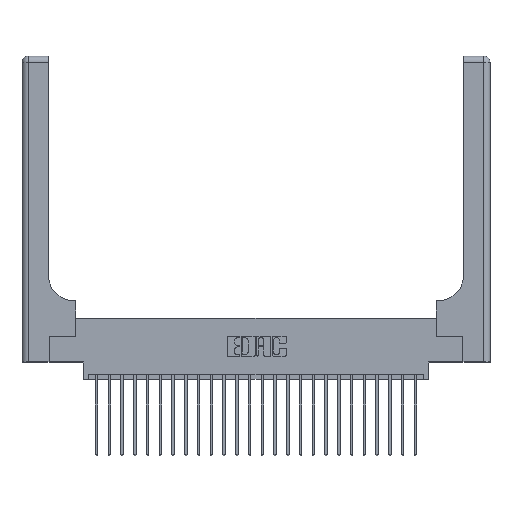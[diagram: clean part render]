
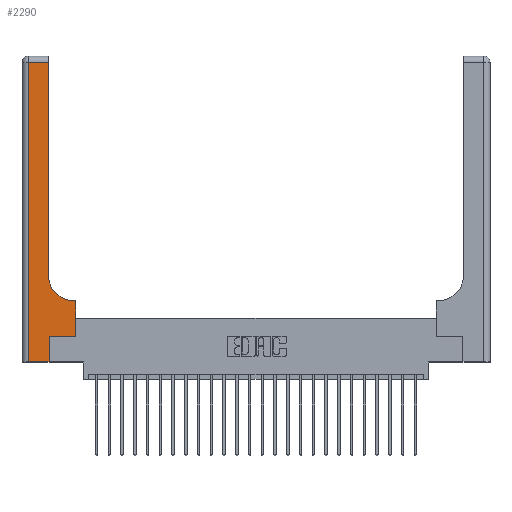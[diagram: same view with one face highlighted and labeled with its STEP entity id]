
A CAD part, top view. The second image highlights one B-rep face of the part: STEP entity #2290.
In plain terms, the highlighted planar face has unit normal (0, 0, 1).
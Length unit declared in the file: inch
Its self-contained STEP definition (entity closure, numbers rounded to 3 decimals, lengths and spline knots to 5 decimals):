
#198 = DIRECTION ( 'NONE',  ( 1., 0., 0. ) ) ;
#239 = EDGE_CURVE ( 'NONE', #23521, #16799, #15904, .T. ) ;
#291 = EDGE_LOOP ( 'NONE', ( #4478, #24592, #1871, #3739, #15681, #24732, #485, #9673, #7889 ) ) ;
#323 = CARTESIAN_POINT ( 'NONE',  ( 0.528, 0.25, 0.37 ) ) ;
#444 = DIRECTION ( 'NONE',  ( -1., 0., 0. ) ) ;
#485 = ORIENTED_EDGE ( 'NONE', *, *, #17628, .T. ) ;
#491 = VECTOR ( 'NONE', #2078, 39.37008 ) ;
#768 = VERTEX_POINT ( 'NONE', #23252 ) ;
#854 = VERTEX_POINT ( 'NONE', #15691 ) ;
#862 = VECTOR ( 'NONE', #1539, 39.37008 ) ;
#1539 = DIRECTION ( 'NONE',  ( 0., 1., 0. ) ) ;
#1871 = ORIENTED_EDGE ( 'NONE', *, *, #14833, .T. ) ;
#2078 = DIRECTION ( 'NONE',  ( -1., 0., 0. ) ) ;
#2208 = CARTESIAN_POINT ( 'NONE',  ( 0.26, 0.6, 0.37 ) ) ;
#2290 = ADVANCED_FACE ( 'NONE', ( #17713 ), #2577, .F. ) ;
#2577 = PLANE ( 'NONE',  #14267 ) ;
#2630 = DIRECTION ( 'NONE',  ( 0., 1., 0. ) ) ;
#2984 = VECTOR ( 'NONE', #18161, 39.37008 ) ;
#3313 = VERTEX_POINT ( 'NONE', #3634 ) ;
#3634 = CARTESIAN_POINT ( 'NONE',  ( 0.26, 2.94, 0.37 ) ) ;
#3709 = CARTESIAN_POINT ( 'NONE',  ( 0.265, 0., 0.37 ) ) ;
#3739 = ORIENTED_EDGE ( 'NONE', *, *, #14933, .T. ) ;
#3963 = VERTEX_POINT ( 'NONE', #13200 ) ;
#3987 = DIRECTION ( 'NONE',  ( 0., 0., -1. ) ) ;
#4138 = EDGE_CURVE ( 'NONE', #13338, #23521, #16810, .T. ) ;
#4478 = ORIENTED_EDGE ( 'NONE', *, *, #21760, .T. ) ;
#4628 = VERTEX_POINT ( 'NONE', #5416 ) ;
#5118 = EDGE_CURVE ( 'NONE', #854, #22644, #17482, .T. ) ;
#5131 = EDGE_CURVE ( 'NONE', #3313, #4628, #15595, .T. ) ;
#5416 = CARTESIAN_POINT ( 'NONE',  ( 0.06, 2.94, 0.37 ) ) ;
#5643 = CARTESIAN_POINT ( 'NONE',  ( 0.06, 3., 0.37 ) ) ;
#5755 = CARTESIAN_POINT ( 'NONE',  ( 0., 2.94, 0.37 ) ) ;
#6019 = CARTESIAN_POINT ( 'NONE',  ( 0., 0., 0.37 ) ) ;
#6179 = AXIS2_PLACEMENT_3D ( 'NONE', #12033, #23136, #198 ) ;
#7767 = DIRECTION ( 'NONE',  ( 1., 0., 0. ) ) ;
#7889 = ORIENTED_EDGE ( 'NONE', *, *, #22167, .T. ) ;
#8161 = VECTOR ( 'NONE', #8395, 39.37008 ) ;
#8395 = DIRECTION ( 'NONE',  ( 0., 1., 0. ) ) ;
#8538 = LINE ( 'NONE', #19910, #23062 ) ;
#8716 = LINE ( 'NONE', #6019, #21770 ) ;
#8886 = VECTOR ( 'NONE', #24309, 39.37008 ) ;
#9673 = ORIENTED_EDGE ( 'NONE', *, *, #5118, .T. ) ;
#11314 = LINE ( 'NONE', #5643, #8886 ) ;
#12033 = CARTESIAN_POINT ( 'NONE',  ( 0.51, 0.85, 0.37 ) ) ;
#13200 = CARTESIAN_POINT ( 'NONE',  ( 0.26, 0.85, 0.37 ) ) ;
#13338 = VERTEX_POINT ( 'NONE', #3709 ) ;
#13553 = CARTESIAN_POINT ( 'NONE',  ( 0., 3., 0.37 ) ) ;
#14003 = CARTESIAN_POINT ( 'NONE',  ( 0.265, 0.25, 0.37 ) ) ;
#14267 = AXIS2_PLACEMENT_3D ( 'NONE', #13553, #3987, #444 ) ;
#14833 = EDGE_CURVE ( 'NONE', #4628, #768, #11314, .T. ) ;
#14933 = EDGE_CURVE ( 'NONE', #768, #13338, #8716, .T. ) ;
#15595 = LINE ( 'NONE', #5755, #16210 ) ;
#15681 = ORIENTED_EDGE ( 'NONE', *, *, #4138, .T. ) ;
#15691 = CARTESIAN_POINT ( 'NONE',  ( 0.528, 0.6, 0.37 ) ) ;
#15904 = LINE ( 'NONE', #14003, #2984 ) ;
#16210 = VECTOR ( 'NONE', #21137, 39.37008 ) ;
#16799 = VERTEX_POINT ( 'NONE', #323 ) ;
#16810 = LINE ( 'NONE', #18818, #862 ) ;
#17482 = LINE ( 'NONE', #2208, #491 ) ;
#17628 = EDGE_CURVE ( 'NONE', #16799, #854, #8538, .T. ) ;
#17713 = FACE_OUTER_BOUND ( 'NONE', #291, .T. ) ;
#18161 = DIRECTION ( 'NONE',  ( 1., 0., 0. ) ) ;
#18262 = CIRCLE ( 'NONE', #6179, 0.25 ) ;
#18818 = CARTESIAN_POINT ( 'NONE',  ( 0.265, 0., 0.37 ) ) ;
#19479 = CARTESIAN_POINT ( 'NONE',  ( 0.265, 0.25, 0.37 ) ) ;
#19910 = CARTESIAN_POINT ( 'NONE',  ( 0.528, 0.25, 0.37 ) ) ;
#20258 = LINE ( 'NONE', #22393, #8161 ) ;
#21137 = DIRECTION ( 'NONE',  ( -1., 0., 0. ) ) ;
#21213 = CARTESIAN_POINT ( 'NONE',  ( 0.51, 0.6, 0.37 ) ) ;
#21760 = EDGE_CURVE ( 'NONE', #3963, #3313, #20258, .T. ) ;
#21770 = VECTOR ( 'NONE', #7767, 39.37008 ) ;
#22167 = EDGE_CURVE ( 'NONE', #22644, #3963, #18262, .T. ) ;
#22393 = CARTESIAN_POINT ( 'NONE',  ( 0.26, 3., 0.37 ) ) ;
#22644 = VERTEX_POINT ( 'NONE', #21213 ) ;
#23062 = VECTOR ( 'NONE', #2630, 39.37008 ) ;
#23136 = DIRECTION ( 'NONE',  ( 0., 0., -1. ) ) ;
#23252 = CARTESIAN_POINT ( 'NONE',  ( 0.06, 0., 0.37 ) ) ;
#23521 = VERTEX_POINT ( 'NONE', #19479 ) ;
#24309 = DIRECTION ( 'NONE',  ( 0., -1., 0. ) ) ;
#24592 = ORIENTED_EDGE ( 'NONE', *, *, #5131, .T. ) ;
#24732 = ORIENTED_EDGE ( 'NONE', *, *, #239, .T. ) ;
